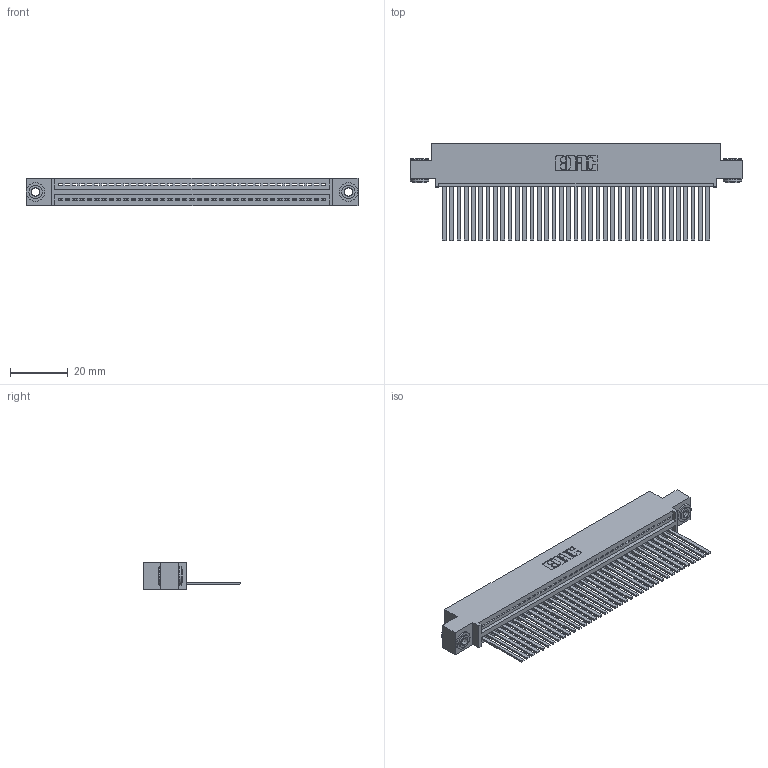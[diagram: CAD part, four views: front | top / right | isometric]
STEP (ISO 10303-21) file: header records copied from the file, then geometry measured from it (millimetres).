
FILE_DESCRIPTION (( 'STEP AP203' ), '1' );
FILE_NAME ('395-037-544-403.STEP', '2018-11-14T00:20:10', ( '' ), ( '' ), 'SwSTEP 2.0', 'SolidWorks 2016', '' );
FILE_SCHEMA (( 'CONFIG_CONTROL_DESIGN' ));
Length unit declared in the file: inch
Products named in the file (4): 395-037-544-403; 345-292-001_345-293-144; 345 Part_0.110 Offset - 0.156 Dia-TH; 345-250-002_345-250-002-102
Assembly tree (40 placements, depth 2):
  395-037-544-403
    345 Part_0.110 Offset - 0.156 Dia-TH
    345-292-001_345-293-144  x37
    345-250-002_345-250-002-102  x2
Bounding box: 115.19 x 33.96 x 9.4 mm (x, y, z)
Volume: 11274.3 mm3; surface area: 16497.4 mm2
Topology: 40 solids, 40 shells, 2092 faces, 6275 edges, 4130 vertices
Faces by surface type: plane 1426, cylinder 658, cone 8
Entity records: 29118 total; most frequent: CARTESIAN_POINT 5022, ORIENTED_EDGE 4986, DIRECTION 4421, EDGE_CURVE 2493, VECTOR 2193, LINE 2193, VERTEX_POINT 1658, AXIS2_PLACEMENT_3D 1114
